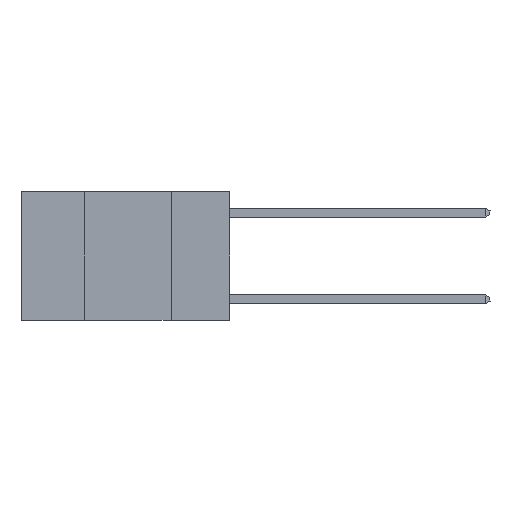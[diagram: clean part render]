
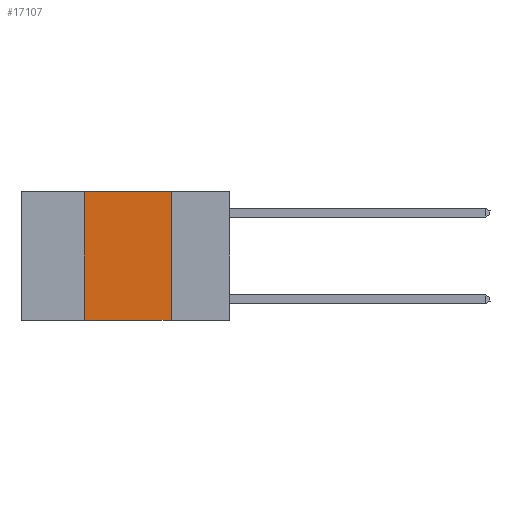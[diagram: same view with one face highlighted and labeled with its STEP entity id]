
A CAD part, left-side view. The second image highlights one B-rep face of the part: STEP entity #17107.
In plain terms, the highlighted planar face has unit normal (-1, 0, 0).
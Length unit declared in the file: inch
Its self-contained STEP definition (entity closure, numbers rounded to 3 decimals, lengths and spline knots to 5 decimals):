
#617 = LINE ( 'NONE', #13859, #1549 ) ;
#1029 = VERTEX_POINT ( 'NONE', #25845 ) ;
#1123 = ORIENTED_EDGE ( 'NONE', *, *, #13078, .F. ) ;
#1549 = VECTOR ( 'NONE', #20753, 39.37008 ) ;
#2735 = EDGE_LOOP ( 'NONE', ( #4883, #1123, #26314, #17556 ) ) ;
#3328 = CARTESIAN_POINT ( 'NONE',  ( 0., 0.6, -0.37 ) ) ;
#4165 = CARTESIAN_POINT ( 'NONE',  ( 0., 0.17, 0. ) ) ;
#4883 = ORIENTED_EDGE ( 'NONE', *, *, #12002, .F. ) ;
#5984 = CARTESIAN_POINT ( 'NONE',  ( 0., 0.6, 0. ) ) ;
#8218 = VERTEX_POINT ( 'NONE', #4165 ) ;
#8733 = LINE ( 'NONE', #18002, #27389 ) ;
#10524 = FACE_OUTER_BOUND ( 'NONE', #2735, .T. ) ;
#12002 = EDGE_CURVE ( 'NONE', #8218, #19037, #617, .T. ) ;
#12003 = DIRECTION ( 'NONE',  ( 0., -1., 0. ) ) ;
#12371 = VERTEX_POINT ( 'NONE', #25969 ) ;
#13078 = EDGE_CURVE ( 'NONE', #12371, #8218, #8733, .T. ) ;
#13859 = CARTESIAN_POINT ( 'NONE',  ( 0., 0.17, 0. ) ) ;
#14890 = DIRECTION ( 'NONE',  ( 0., 0., 1. ) ) ;
#14939 = DIRECTION ( 'NONE',  ( 0., 0., -1. ) ) ;
#15531 = DIRECTION ( 'NONE',  ( 1., 0., 0. ) ) ;
#16358 = VECTOR ( 'NONE', #14890, 39.37008 ) ;
#17000 = EDGE_CURVE ( 'NONE', #1029, #19037, #27753, .T. ) ;
#17107 = ADVANCED_FACE ( 'NONE', ( #10524 ), #26271, .F. ) ;
#17556 = ORIENTED_EDGE ( 'NONE', *, *, #17000, .T. ) ;
#17709 = DIRECTION ( 'NONE',  ( 0., -1., 0. ) ) ;
#18002 = CARTESIAN_POINT ( 'NONE',  ( 0., 0.6, 0. ) ) ;
#19037 = VERTEX_POINT ( 'NONE', #28027 ) ;
#20753 = DIRECTION ( 'NONE',  ( 0., 0., -1. ) ) ;
#20819 = LINE ( 'NONE', #26224, #16358 ) ;
#24242 = AXIS2_PLACEMENT_3D ( 'NONE', #5984, #15531, #14939 ) ;
#25458 = EDGE_CURVE ( 'NONE', #1029, #12371, #20819, .T. ) ;
#25845 = CARTESIAN_POINT ( 'NONE',  ( 0., 0.42, -0.37 ) ) ;
#25969 = CARTESIAN_POINT ( 'NONE',  ( 0., 0.42, 0. ) ) ;
#26224 = CARTESIAN_POINT ( 'NONE',  ( 0., 0.42, 0. ) ) ;
#26271 = PLANE ( 'NONE',  #24242 ) ;
#26314 = ORIENTED_EDGE ( 'NONE', *, *, #25458, .F. ) ;
#27389 = VECTOR ( 'NONE', #17709, 39.37008 ) ;
#27753 = LINE ( 'NONE', #3328, #28001 ) ;
#28001 = VECTOR ( 'NONE', #12003, 39.37008 ) ;
#28027 = CARTESIAN_POINT ( 'NONE',  ( 0., 0.17, -0.37 ) ) ;
